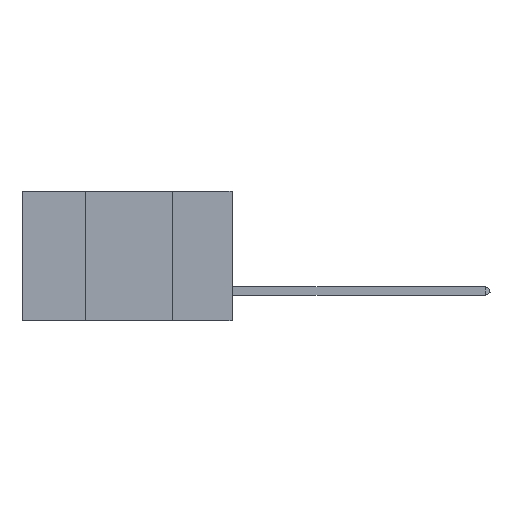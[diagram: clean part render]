
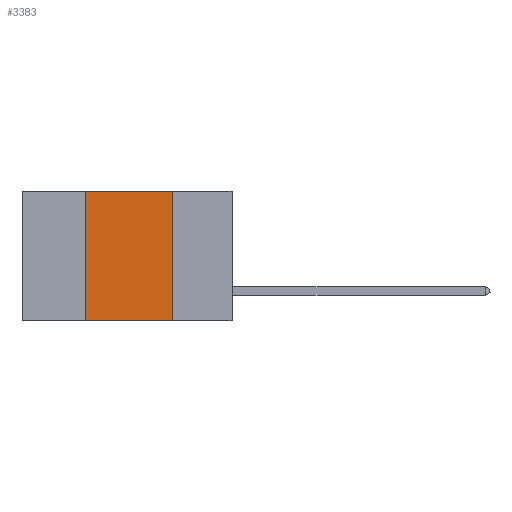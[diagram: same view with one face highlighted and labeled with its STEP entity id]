
A CAD part, left-side view. The second image highlights one B-rep face of the part: STEP entity #3383.
In plain terms, the highlighted planar face has unit normal (-1, 0, 0).
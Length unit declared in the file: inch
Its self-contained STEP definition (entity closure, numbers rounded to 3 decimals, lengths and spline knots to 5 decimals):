
#256 = DIRECTION ( 'NONE',  ( 0., 0., 1. ) ) ;
#760 = FACE_OUTER_BOUND ( 'NONE', #9081, .T. ) ;
#1500 = LINE ( 'NONE', #7534, #6225 ) ;
#1631 = ORIENTED_EDGE ( 'NONE', *, *, #5081, .T. ) ;
#1836 = VERTEX_POINT ( 'NONE', #9602 ) ;
#2433 = CARTESIAN_POINT ( 'NONE',  ( 0., 0.6, -0.37 ) ) ;
#3383 = ADVANCED_FACE ( 'NONE', ( #760 ), #4992, .F. ) ;
#4747 = CARTESIAN_POINT ( 'NONE',  ( 0., 0.17, 0. ) ) ;
#4868 = VERTEX_POINT ( 'NONE', #16378 ) ;
#4992 = PLANE ( 'NONE',  #19098 ) ;
#5081 = EDGE_CURVE ( 'NONE', #1836, #13458, #12793, .T. ) ;
#6225 = VECTOR ( 'NONE', #16437, 39.37008 ) ;
#6638 = ORIENTED_EDGE ( 'NONE', *, *, #21246, .F. ) ;
#7534 = CARTESIAN_POINT ( 'NONE',  ( 0., 0.17, 0. ) ) ;
#7779 = ORIENTED_EDGE ( 'NONE', *, *, #8561, .F. ) ;
#8528 = CARTESIAN_POINT ( 'NONE',  ( 0., 0.6, 0. ) ) ;
#8561 = EDGE_CURVE ( 'NONE', #1836, #4868, #15021, .T. ) ;
#9081 = EDGE_LOOP ( 'NONE', ( #14220, #6638, #7779, #1631 ) ) ;
#9602 = CARTESIAN_POINT ( 'NONE',  ( 0., 0.42, -0.37 ) ) ;
#10052 = EDGE_CURVE ( 'NONE', #11177, #13458, #1500, .T. ) ;
#10288 = DIRECTION ( 'NONE',  ( 0., 0., -1. ) ) ;
#10448 = CARTESIAN_POINT ( 'NONE',  ( 0., 0.42, 0. ) ) ;
#10514 = VECTOR ( 'NONE', #256, 39.37008 ) ;
#11177 = VERTEX_POINT ( 'NONE', #4747 ) ;
#12793 = LINE ( 'NONE', #2433, #20424 ) ;
#13207 = CARTESIAN_POINT ( 'NONE',  ( 0., 0.6, 0. ) ) ;
#13458 = VERTEX_POINT ( 'NONE', #21017 ) ;
#13771 = DIRECTION ( 'NONE',  ( 0., -1., 0. ) ) ;
#14220 = ORIENTED_EDGE ( 'NONE', *, *, #10052, .F. ) ;
#14411 = LINE ( 'NONE', #13207, #18357 ) ;
#15021 = LINE ( 'NONE', #10448, #10514 ) ;
#15379 = DIRECTION ( 'NONE',  ( 1., 0., 0. ) ) ;
#16378 = CARTESIAN_POINT ( 'NONE',  ( 0., 0.42, 0. ) ) ;
#16437 = DIRECTION ( 'NONE',  ( 0., 0., -1. ) ) ;
#18357 = VECTOR ( 'NONE', #19907, 39.37008 ) ;
#19098 = AXIS2_PLACEMENT_3D ( 'NONE', #8528, #15379, #10288 ) ;
#19907 = DIRECTION ( 'NONE',  ( 0., -1., 0. ) ) ;
#20424 = VECTOR ( 'NONE', #13771, 39.37008 ) ;
#21017 = CARTESIAN_POINT ( 'NONE',  ( 0., 0.17, -0.37 ) ) ;
#21246 = EDGE_CURVE ( 'NONE', #4868, #11177, #14411, .T. ) ;
